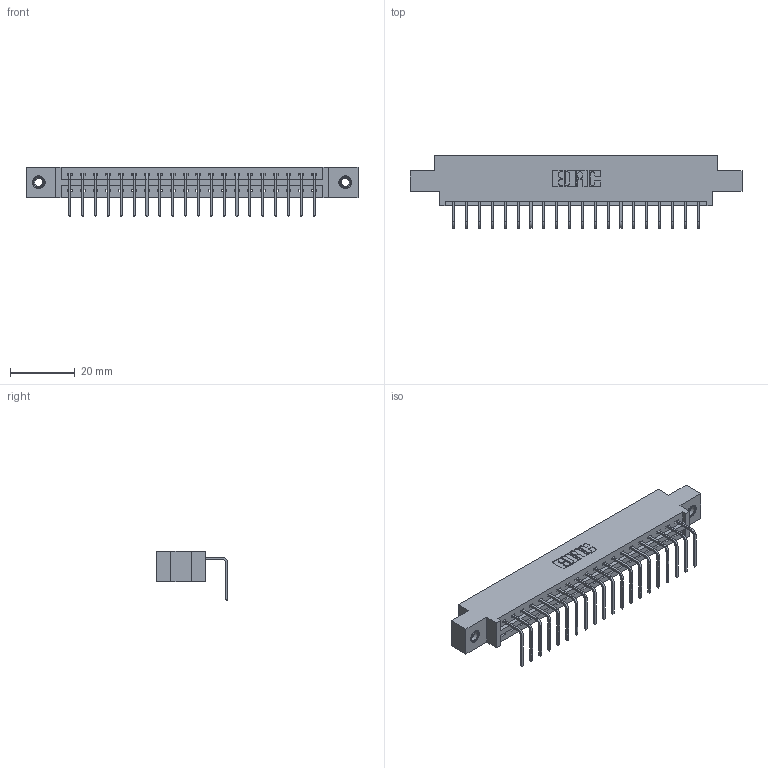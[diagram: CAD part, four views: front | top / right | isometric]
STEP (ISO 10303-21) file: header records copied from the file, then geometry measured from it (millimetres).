
FILE_DESCRIPTION (( 'STEP AP203' ), '1' );
FILE_NAME ('387-020-558-607.STEP', '2018-09-14T00:25:15', ( '' ), ( '' ), 'SwSTEP 2.0', 'SolidWorks 2016', '' );
FILE_SCHEMA (( 'CONFIG_CONTROL_DESIGN' ));
Length unit declared in the file: inch
Products named in the file (4): 345-292-001_558 Tail - 2; 345-250-001_345-250-005-103; 387-020-558-607; 337 Part_0.170 Offset - 0.156 Dia-TI
Assembly tree (23 placements, depth 2):
  387-020-558-607
    337 Part_0.170 Offset - 0.156 Dia-TI
    345-292-001_558 Tail - 2  x20
    345-250-001_345-250-005-103  x2
Bounding box: 102.26 x 22.17 x 15.37 mm (x, y, z)
Volume: 10288.6 mm3; surface area: 11056.5 mm2
Topology: 23 solids, 23 shells, 1458 faces, 4339 edges, 2858 vertices
Faces by surface type: plane 1066, cylinder 376, cone 12, torus 4
Entity records: 19114 total; most frequent: CARTESIAN_POINT 3309, ORIENTED_EDGE 3258, DIRECTION 2863, EDGE_CURVE 1629, LINE 1481, VECTOR 1481, VERTEX_POINT 1080, AXIS2_PLACEMENT_3D 691
